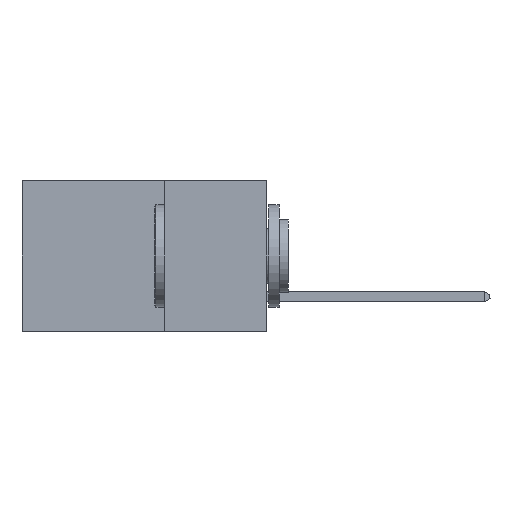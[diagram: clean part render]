
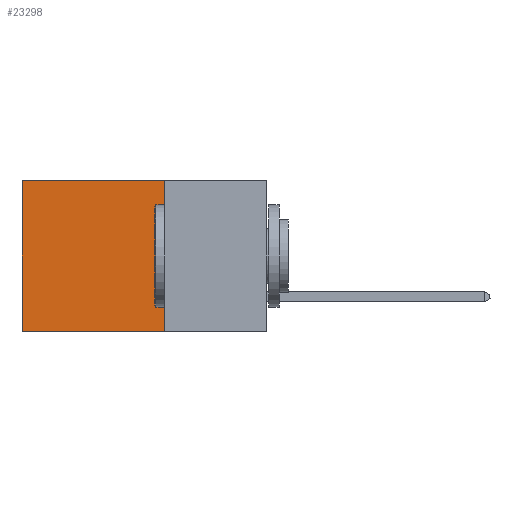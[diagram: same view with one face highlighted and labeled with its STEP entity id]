
A CAD part, left-side view. The second image highlights one B-rep face of the part: STEP entity #23298.
In plain terms, the highlighted planar face has unit normal (-1, 0, 0).
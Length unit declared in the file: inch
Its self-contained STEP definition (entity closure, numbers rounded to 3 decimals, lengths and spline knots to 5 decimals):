
#1129 = VECTOR ( 'NONE', #8607, 39.37008 ) ;
#1844 = DIRECTION ( 'NONE',  ( 0., 0., -1. ) ) ;
#2664 = PLANE ( 'NONE',  #39018 ) ;
#2809 = VERTEX_POINT ( 'NONE', #8186 ) ;
#3439 = VERTEX_POINT ( 'NONE', #32644 ) ;
#3633 = CARTESIAN_POINT ( 'NONE',  ( 0.2875, 0.6, 0. ) ) ;
#4819 = EDGE_LOOP ( 'NONE', ( #7112, #37810, #10867, #14464 ) ) ;
#6638 = CARTESIAN_POINT ( 'NONE',  ( 0.2875, 0.25, -0.37 ) ) ;
#6767 = DIRECTION ( 'NONE',  ( 0., 1., 0. ) ) ;
#7112 = ORIENTED_EDGE ( 'NONE', *, *, #14997, .T. ) ;
#8186 = CARTESIAN_POINT ( 'NONE',  ( 0.2875, 0.25, -0.37 ) ) ;
#8607 = DIRECTION ( 'NONE',  ( 0., 1., 0. ) ) ;
#8889 = CARTESIAN_POINT ( 'NONE',  ( 0.2875, 0.25, 0. ) ) ;
#9181 = LINE ( 'NONE', #10695, #19018 ) ;
#9915 = LINE ( 'NONE', #36789, #19769 ) ;
#10695 = CARTESIAN_POINT ( 'NONE',  ( 0.2875, 0.25, 0. ) ) ;
#10867 = ORIENTED_EDGE ( 'NONE', *, *, #19036, .F. ) ;
#11202 = VERTEX_POINT ( 'NONE', #3633 ) ;
#12928 = LINE ( 'NONE', #8889, #1129 ) ;
#14376 = DIRECTION ( 'NONE',  ( 1., 0., 0. ) ) ;
#14464 = ORIENTED_EDGE ( 'NONE', *, *, #32086, .T. ) ;
#14997 = EDGE_CURVE ( 'NONE', #11202, #18998, #9915, .T. ) ;
#18897 = DIRECTION ( 'NONE',  ( 0., 0., -1. ) ) ;
#18998 = VERTEX_POINT ( 'NONE', #21127 ) ;
#19018 = VECTOR ( 'NONE', #1844, 39.37008 ) ;
#19036 = EDGE_CURVE ( 'NONE', #3439, #2809, #9181, .T. ) ;
#19769 = VECTOR ( 'NONE', #18897, 39.37008 ) ;
#21127 = CARTESIAN_POINT ( 'NONE',  ( 0.2875, 0.6, -0.37 ) ) ;
#23298 = ADVANCED_FACE ( 'NONE', ( #26008 ), #2664, .F. ) ;
#23905 = VECTOR ( 'NONE', #6767, 39.37008 ) ;
#26008 = FACE_OUTER_BOUND ( 'NONE', #4819, .T. ) ;
#26871 = DIRECTION ( 'NONE',  ( 0., 0., -1. ) ) ;
#31911 = LINE ( 'NONE', #6638, #23905 ) ;
#32086 = EDGE_CURVE ( 'NONE', #3439, #11202, #12928, .T. ) ;
#32644 = CARTESIAN_POINT ( 'NONE',  ( 0.2875, 0.25, 0. ) ) ;
#35611 = CARTESIAN_POINT ( 'NONE',  ( 0.2875, 0.25, 0. ) ) ;
#36789 = CARTESIAN_POINT ( 'NONE',  ( 0.2875, 0.6, 0. ) ) ;
#37326 = EDGE_CURVE ( 'NONE', #2809, #18998, #31911, .T. ) ;
#37810 = ORIENTED_EDGE ( 'NONE', *, *, #37326, .F. ) ;
#39018 = AXIS2_PLACEMENT_3D ( 'NONE', #35611, #14376, #26871 ) ;
